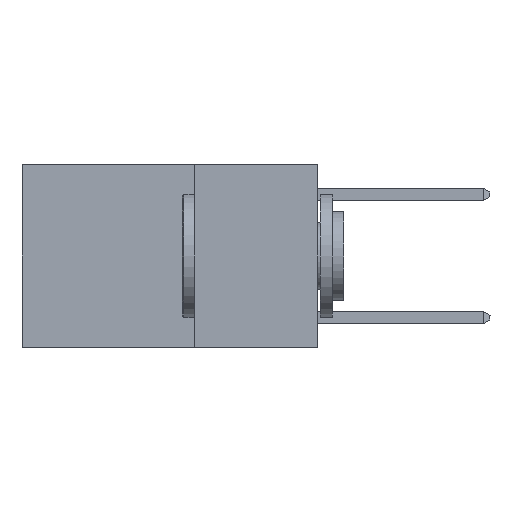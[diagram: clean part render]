
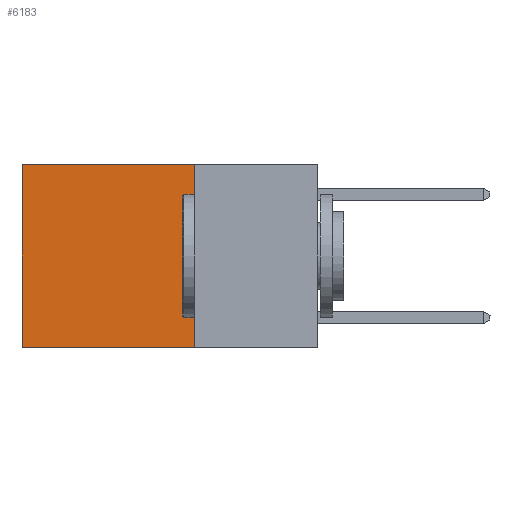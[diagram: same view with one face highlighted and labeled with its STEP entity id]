
A CAD part, left-side view. The second image highlights one B-rep face of the part: STEP entity #6183.
In plain terms, the highlighted planar face has unit normal (-1, 0, 0).
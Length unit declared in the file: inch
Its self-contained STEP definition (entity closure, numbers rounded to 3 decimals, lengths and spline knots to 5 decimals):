
#524 = EDGE_CURVE ( 'NONE', #3853, #5303, #7205, .T. ) ;
#1566 = VERTEX_POINT ( 'NONE', #5558 ) ;
#1655 = CARTESIAN_POINT ( 'NONE',  ( 0.2625, 0.25, -0.37 ) ) ;
#1730 = EDGE_LOOP ( 'NONE', ( #6910, #8024, #8122, #8317 ) ) ;
#1898 = CARTESIAN_POINT ( 'NONE',  ( 0.2625, 0.25, 0. ) ) ;
#1918 = CARTESIAN_POINT ( 'NONE',  ( 0.2625, 0.6, 0. ) ) ;
#2398 = LINE ( 'NONE', #1898, #8513 ) ;
#2565 = CARTESIAN_POINT ( 'NONE',  ( 0.2625, 0.25, 0. ) ) ;
#3041 = CARTESIAN_POINT ( 'NONE',  ( 0.2625, 0.6, -0.37 ) ) ;
#3428 = DIRECTION ( 'NONE',  ( 0., 0., -1. ) ) ;
#3448 = CARTESIAN_POINT ( 'NONE',  ( 0.2625, 0.25, 0. ) ) ;
#3853 = VERTEX_POINT ( 'NONE', #1655 ) ;
#4444 = DIRECTION ( 'NONE',  ( 0., 0., -1. ) ) ;
#4839 = VECTOR ( 'NONE', #6367, 39.37008 ) ;
#4896 = AXIS2_PLACEMENT_3D ( 'NONE', #2565, #8178, #3428 ) ;
#5137 = FACE_OUTER_BOUND ( 'NONE', #1730, .T. ) ;
#5303 = VERTEX_POINT ( 'NONE', #3041 ) ;
#5558 = CARTESIAN_POINT ( 'NONE',  ( 0.2625, 0.25, 0. ) ) ;
#5690 = EDGE_CURVE ( 'NONE', #8736, #5303, #8301, .T. ) ;
#5781 = CARTESIAN_POINT ( 'NONE',  ( 0.2625, 0.6, 0. ) ) ;
#6183 = ADVANCED_FACE ( 'NONE', ( #5137 ), #7420, .F. ) ;
#6298 = VECTOR ( 'NONE', #4444, 39.37008 ) ;
#6367 = DIRECTION ( 'NONE',  ( 0., 1., 0. ) ) ;
#6517 = VECTOR ( 'NONE', #8910, 39.37008 ) ;
#6910 = ORIENTED_EDGE ( 'NONE', *, *, #5690, .T. ) ;
#7205 = LINE ( 'NONE', #9768, #4839 ) ;
#7420 = PLANE ( 'NONE',  #4896 ) ;
#7592 = DIRECTION ( 'NONE',  ( 0., 1., 0. ) ) ;
#8024 = ORIENTED_EDGE ( 'NONE', *, *, #524, .F. ) ;
#8122 = ORIENTED_EDGE ( 'NONE', *, *, #9754, .F. ) ;
#8178 = DIRECTION ( 'NONE',  ( 1., 0., 0. ) ) ;
#8301 = LINE ( 'NONE', #1918, #6298 ) ;
#8317 = ORIENTED_EDGE ( 'NONE', *, *, #9109, .T. ) ;
#8506 = LINE ( 'NONE', #3448, #6517 ) ;
#8513 = VECTOR ( 'NONE', #7592, 39.37008 ) ;
#8736 = VERTEX_POINT ( 'NONE', #5781 ) ;
#8910 = DIRECTION ( 'NONE',  ( 0., 0., -1. ) ) ;
#9109 = EDGE_CURVE ( 'NONE', #1566, #8736, #2398, .T. ) ;
#9754 = EDGE_CURVE ( 'NONE', #1566, #3853, #8506, .T. ) ;
#9768 = CARTESIAN_POINT ( 'NONE',  ( 0.2625, 0.25, -0.37 ) ) ;
